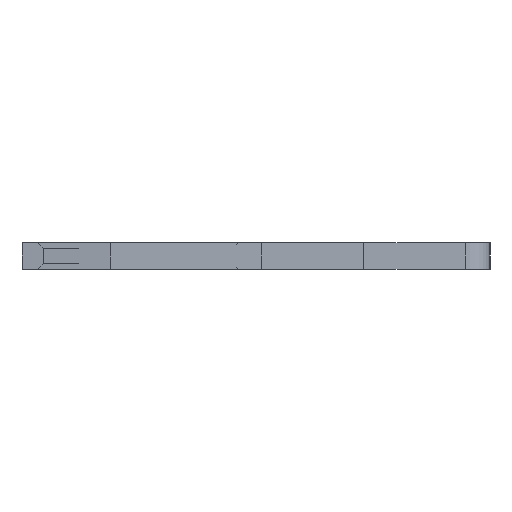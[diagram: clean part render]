
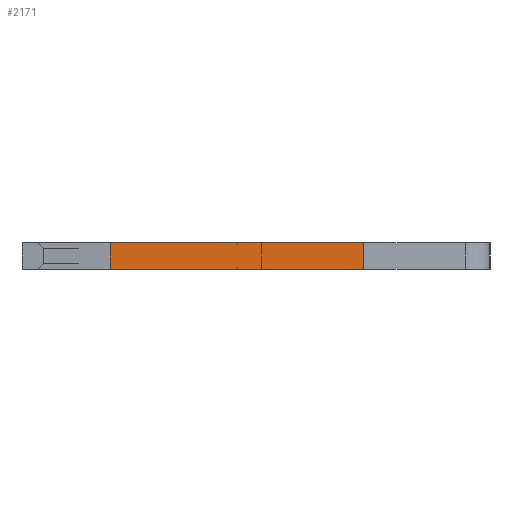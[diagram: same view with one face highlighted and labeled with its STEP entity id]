
A CAD part, left-side view. The second image highlights one B-rep face of the part: STEP entity #2171.
In plain terms, the highlighted face is planar.
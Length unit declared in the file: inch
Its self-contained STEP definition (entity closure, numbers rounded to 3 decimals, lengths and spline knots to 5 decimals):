
#70 = EDGE_CURVE ( 'NONE', #2341, #483, #303, .T. ) ;
#91 = DIRECTION ( 'NONE',  ( -1., 0., 0. ) ) ;
#117 = FACE_OUTER_BOUND ( 'NONE', #864, .T. ) ;
#201 = ORIENTED_EDGE ( 'NONE', *, *, #2510, .F. ) ;
#303 = LINE ( 'NONE', #314, #338 ) ;
#312 = AXIS2_PLACEMENT_3D ( 'NONE', #1082, #2417, #1074 ) ;
#314 = CARTESIAN_POINT ( 'NONE',  ( 0.013, -0.099, -0.0575 ) ) ;
#338 = VECTOR ( 'NONE', #91, 39.37008 ) ;
#343 = VECTOR ( 'NONE', #2402, 39.37008 ) ;
#378 = CARTESIAN_POINT ( 'NONE',  ( -0.013, -0.099, -0.0575 ) ) ;
#467 = DIRECTION ( 'NONE',  ( -1., 0., 0. ) ) ;
#479 = EDGE_CURVE ( 'NONE', #2341, #2670, #1448, .T. ) ;
#483 = VERTEX_POINT ( 'NONE', #378 ) ;
#709 = DIRECTION ( 'NONE',  ( 0., 1., 0. ) ) ;
#864 = EDGE_LOOP ( 'NONE', ( #1529, #201, #1323, #2704 ) ) ;
#890 = CARTESIAN_POINT ( 'NONE',  ( 0.013, 0.146, -0.0575 ) ) ;
#939 = LINE ( 'NONE', #2249, #2703 ) ;
#981 = EDGE_CURVE ( 'NONE', #483, #2293, #939, .T. ) ;
#1074 = DIRECTION ( 'NONE',  ( 1., 0., 0. ) ) ;
#1082 = CARTESIAN_POINT ( 'NONE',  ( 0.013, 0.146, -0.0575 ) ) ;
#1088 = LINE ( 'NONE', #890, #1190 ) ;
#1190 = VECTOR ( 'NONE', #467, 39.37008 ) ;
#1289 = PLANE ( 'NONE',  #312 ) ;
#1312 = CARTESIAN_POINT ( 'NONE',  ( 0.013, -0.099, -0.0575 ) ) ;
#1323 = ORIENTED_EDGE ( 'NONE', *, *, #479, .F. ) ;
#1448 = LINE ( 'NONE', #2411, #343 ) ;
#1529 = ORIENTED_EDGE ( 'NONE', *, *, #981, .T. ) ;
#1996 = CARTESIAN_POINT ( 'NONE',  ( 0.013, 0.146, -0.0575 ) ) ;
#2171 = ADVANCED_FACE ( 'NONE', ( #117 ), #1289, .F. ) ;
#2249 = CARTESIAN_POINT ( 'NONE',  ( -0.013, 0.146, -0.0575 ) ) ;
#2293 = VERTEX_POINT ( 'NONE', #2620 ) ;
#2341 = VERTEX_POINT ( 'NONE', #1312 ) ;
#2402 = DIRECTION ( 'NONE',  ( 0., 1., 0. ) ) ;
#2411 = CARTESIAN_POINT ( 'NONE',  ( 0.013, 0.146, -0.0575 ) ) ;
#2417 = DIRECTION ( 'NONE',  ( 0., 0., 1. ) ) ;
#2510 = EDGE_CURVE ( 'NONE', #2670, #2293, #1088, .T. ) ;
#2620 = CARTESIAN_POINT ( 'NONE',  ( -0.013, 0.146, -0.0575 ) ) ;
#2670 = VERTEX_POINT ( 'NONE', #1996 ) ;
#2703 = VECTOR ( 'NONE', #709, 39.37008 ) ;
#2704 = ORIENTED_EDGE ( 'NONE', *, *, #70, .T. ) ;
